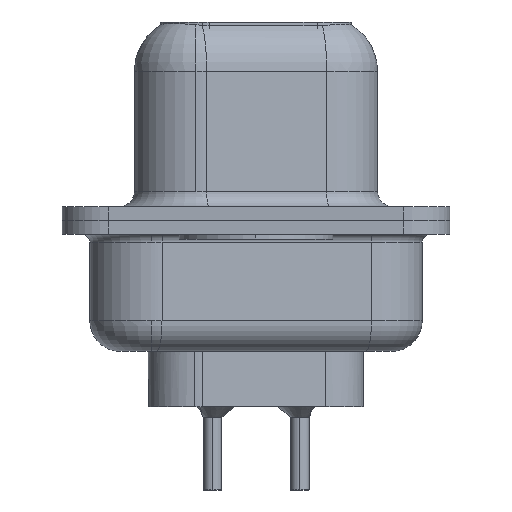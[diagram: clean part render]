
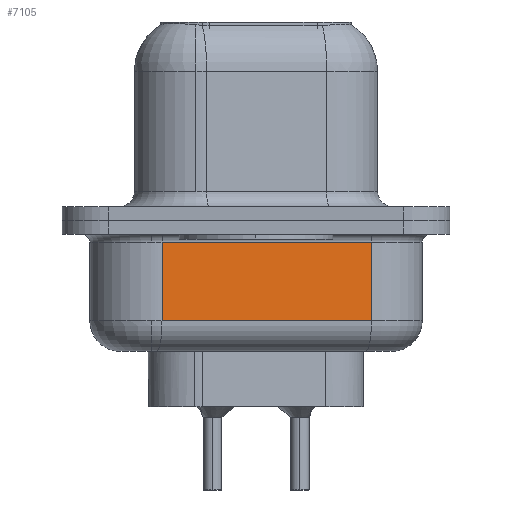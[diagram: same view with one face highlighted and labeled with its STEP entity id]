
A CAD part, left-side view. The second image highlights one B-rep face of the part: STEP entity #7105.
In plain terms, the highlighted planar face has unit normal (-0.985, -0.174, 0).
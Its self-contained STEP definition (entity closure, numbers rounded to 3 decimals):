
#875 = VERTEX_POINT ( 'NONE', #7284 ) ;
#1047 = LINE ( 'NONE', #9461, #5131 ) ;
#2288 = EDGE_CURVE ( 'NONE', #875, #6714, #7244, .T. ) ;
#2377 = CARTESIAN_POINT ( 'NONE',  ( 4.074, -3.747, -3.25 ) ) ;
#2557 = EDGE_CURVE ( 'NONE', #9638, #875, #19231, .T. ) ;
#3137 = CARTESIAN_POINT ( 'NONE',  ( 2.875, 3.053, -4.25 ) ) ;
#3316 = CARTESIAN_POINT ( 'NONE',  ( 2.875, 3.053, -0.7 ) ) ;
#3378 = VECTOR ( 'NONE', #16818, 1000. ) ;
#3457 = EDGE_LOOP ( 'NONE', ( #8877, #18892, #12018, #12557 ) ) ;
#3567 = DIRECTION ( 'NONE',  ( -0.174, 0.985, 0. ) ) ;
#4255 = LINE ( 'NONE', #13994, #6931 ) ;
#4572 = VECTOR ( 'NONE', #3567, 1000. ) ;
#4756 = DIRECTION ( 'NONE',  ( 0., 0., 1. ) ) ;
#5131 = VECTOR ( 'NONE', #15558, 1000. ) ;
#6046 = CARTESIAN_POINT ( 'NONE',  ( 2.875, 3.053, -3.25 ) ) ;
#6209 = DIRECTION ( 'NONE',  ( 0.985, 0.174, 0. ) ) ;
#6714 = VERTEX_POINT ( 'NONE', #14328 ) ;
#6931 = VECTOR ( 'NONE', #4756, 1000. ) ;
#7105 = ADVANCED_FACE ( 'NONE', ( #16998 ), #9272, .F. ) ;
#7244 = LINE ( 'NONE', #3316, #4572 ) ;
#7284 = CARTESIAN_POINT ( 'NONE',  ( 4.074, -3.747, -0.7 ) ) ;
#8032 = AXIS2_PLACEMENT_3D ( 'NONE', #3137, #6209, #17001 ) ;
#8877 = ORIENTED_EDGE ( 'NONE', *, *, #17765, .F. ) ;
#9272 = PLANE ( 'NONE',  #8032 ) ;
#9461 = CARTESIAN_POINT ( 'NONE',  ( 2.875, 3.053, -3.25 ) ) ;
#9638 = VERTEX_POINT ( 'NONE', #2377 ) ;
#10399 = VERTEX_POINT ( 'NONE', #6046 ) ;
#11571 = EDGE_CURVE ( 'NONE', #10399, #9638, #1047, .T. ) ;
#12018 = ORIENTED_EDGE ( 'NONE', *, *, #2557, .T. ) ;
#12557 = ORIENTED_EDGE ( 'NONE', *, *, #2288, .T. ) ;
#13994 = CARTESIAN_POINT ( 'NONE',  ( 2.875, 3.053, -4.25 ) ) ;
#14328 = CARTESIAN_POINT ( 'NONE',  ( 2.875, 3.053, -0.7 ) ) ;
#15558 = DIRECTION ( 'NONE',  ( 0.174, -0.985, 0. ) ) ;
#16818 = DIRECTION ( 'NONE',  ( 0., 0., 1. ) ) ;
#16998 = FACE_OUTER_BOUND ( 'NONE', #3457, .T. ) ;
#17001 = DIRECTION ( 'NONE',  ( -0.174, 0.985, 0. ) ) ;
#17364 = CARTESIAN_POINT ( 'NONE',  ( 4.074, -3.747, -4.25 ) ) ;
#17765 = EDGE_CURVE ( 'NONE', #10399, #6714, #4255, .T. ) ;
#18892 = ORIENTED_EDGE ( 'NONE', *, *, #11571, .T. ) ;
#19231 = LINE ( 'NONE', #17364, #3378 ) ;
